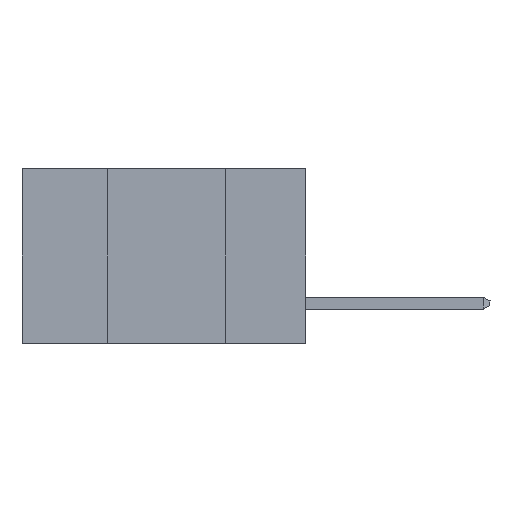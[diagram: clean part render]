
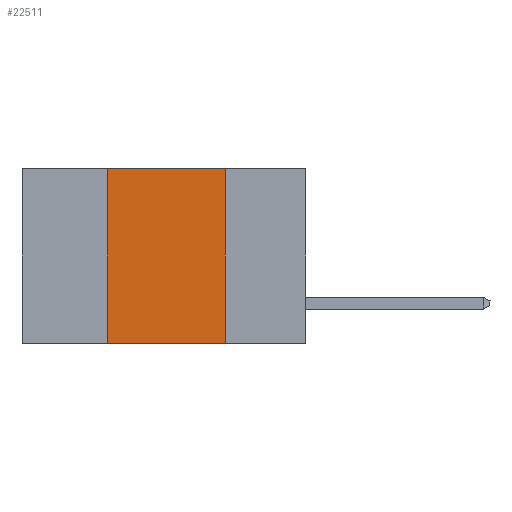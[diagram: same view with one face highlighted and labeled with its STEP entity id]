
A CAD part, left-side view. The second image highlights one B-rep face of the part: STEP entity #22511.
In plain terms, the highlighted planar face has unit normal (-1, 0, 0).
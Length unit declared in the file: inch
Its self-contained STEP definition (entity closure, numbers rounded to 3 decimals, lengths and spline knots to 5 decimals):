
#159 = FACE_OUTER_BOUND ( 'NONE', #16846, .T. ) ;
#274 = EDGE_CURVE ( 'NONE', #3164, #6764, #9465, .T. ) ;
#544 = CARTESIAN_POINT ( 'NONE',  ( 0., 0.17, 0. ) ) ;
#2041 = AXIS2_PLACEMENT_3D ( 'NONE', #9445, #7180, #16460 ) ;
#3164 = VERTEX_POINT ( 'NONE', #544 ) ;
#4249 = LINE ( 'NONE', #17954, #22202 ) ;
#5057 = ORIENTED_EDGE ( 'NONE', *, *, #274, .F. ) ;
#6764 = VERTEX_POINT ( 'NONE', #23464 ) ;
#7180 = DIRECTION ( 'NONE',  ( 1., 0., 0. ) ) ;
#8012 = LINE ( 'NONE', #17164, #18654 ) ;
#8306 = VERTEX_POINT ( 'NONE', #27716 ) ;
#9129 = LINE ( 'NONE', #11458, #29753 ) ;
#9333 = ORIENTED_EDGE ( 'NONE', *, *, #10322, .F. ) ;
#9445 = CARTESIAN_POINT ( 'NONE',  ( 0., 0.6, 0. ) ) ;
#9465 = LINE ( 'NONE', #25772, #28291 ) ;
#9570 = DIRECTION ( 'NONE',  ( 0., 0., 1. ) ) ;
#10322 = EDGE_CURVE ( 'NONE', #8306, #3164, #8012, .T. ) ;
#11076 = CARTESIAN_POINT ( 'NONE',  ( 0., 0.42, -0.37 ) ) ;
#11286 = EDGE_CURVE ( 'NONE', #12710, #6764, #4249, .T. ) ;
#11458 = CARTESIAN_POINT ( 'NONE',  ( 0., 0.42, 0. ) ) ;
#11901 = DIRECTION ( 'NONE',  ( 0., 0., -1. ) ) ;
#12710 = VERTEX_POINT ( 'NONE', #11076 ) ;
#14964 = ORIENTED_EDGE ( 'NONE', *, *, #11286, .T. ) ;
#15971 = DIRECTION ( 'NONE',  ( 0., -1., 0. ) ) ;
#16460 = DIRECTION ( 'NONE',  ( 0., 0., -1. ) ) ;
#16846 = EDGE_LOOP ( 'NONE', ( #5057, #9333, #27215, #14964 ) ) ;
#17164 = CARTESIAN_POINT ( 'NONE',  ( 0., 0.6, 0. ) ) ;
#17954 = CARTESIAN_POINT ( 'NONE',  ( 0., 0.6, -0.37 ) ) ;
#18654 = VECTOR ( 'NONE', #20041, 39.37008 ) ;
#18739 = PLANE ( 'NONE',  #2041 ) ;
#20041 = DIRECTION ( 'NONE',  ( 0., -1., 0. ) ) ;
#22202 = VECTOR ( 'NONE', #15971, 39.37008 ) ;
#22511 = ADVANCED_FACE ( 'NONE', ( #159 ), #18739, .F. ) ;
#23464 = CARTESIAN_POINT ( 'NONE',  ( 0., 0.17, -0.37 ) ) ;
#24175 = EDGE_CURVE ( 'NONE', #12710, #8306, #9129, .T. ) ;
#25772 = CARTESIAN_POINT ( 'NONE',  ( 0., 0.17, 0. ) ) ;
#27215 = ORIENTED_EDGE ( 'NONE', *, *, #24175, .F. ) ;
#27716 = CARTESIAN_POINT ( 'NONE',  ( 0., 0.42, 0. ) ) ;
#28291 = VECTOR ( 'NONE', #11901, 39.37008 ) ;
#29753 = VECTOR ( 'NONE', #9570, 39.37008 ) ;
